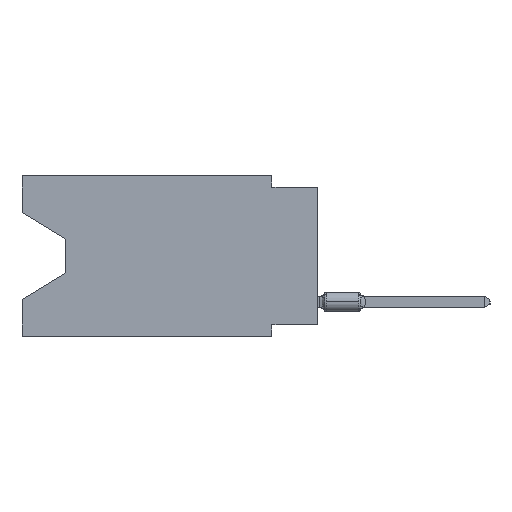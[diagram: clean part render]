
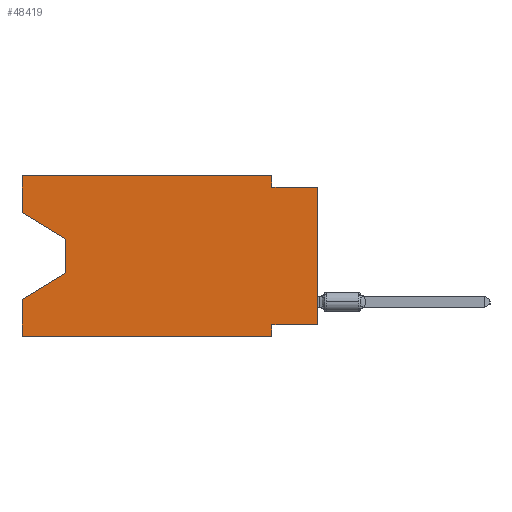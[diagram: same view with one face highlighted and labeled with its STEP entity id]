
A CAD part, left-side view. The second image highlights one B-rep face of the part: STEP entity #48419.
In plain terms, the highlighted planar face has unit normal (-1, 0, 0).
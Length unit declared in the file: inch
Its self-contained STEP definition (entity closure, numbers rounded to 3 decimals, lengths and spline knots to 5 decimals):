
#994 = DIRECTION ( 'NONE',  ( 0., 0., -1. ) ) ;
#1266 = CARTESIAN_POINT ( 'NONE',  ( 0., 0.1, -0.025 ) ) ;
#2979 = LINE ( 'NONE', #18033, #30879 ) ;
#3317 = DIRECTION ( 'NONE',  ( 0., 0.855, -0.519 ) ) ;
#3470 = EDGE_LOOP ( 'NONE', ( #16978, #16556, #7756, #38270, #12181, #52569, #8025, #8264, #33294, #37493, #19391, #17353 ) ) ;
#3641 = EDGE_CURVE ( 'NONE', #18475, #53505, #64559, .T. ) ;
#3717 = CARTESIAN_POINT ( 'NONE',  ( 0., 0.1, 0. ) ) ;
#4876 = CARTESIAN_POINT ( 'NONE',  ( 0., 0.55, -0.138 ) ) ;
#5006 = VECTOR ( 'NONE', #8415, 39.37008 ) ;
#5639 = CARTESIAN_POINT ( 'NONE',  ( 0., 0.645, 0. ) ) ;
#6050 = CARTESIAN_POINT ( 'NONE',  ( 0., 0.645, -0.26975 ) ) ;
#6542 = CARTESIAN_POINT ( 'NONE',  ( 0., 0.645, 0. ) ) ;
#7553 = EDGE_CURVE ( 'NONE', #18475, #38738, #58674, .T. ) ;
#7756 = ORIENTED_EDGE ( 'NONE', *, *, #38244, .T. ) ;
#7978 = EDGE_CURVE ( 'NONE', #9616, #35338, #43878, .T. ) ;
#8025 = ORIENTED_EDGE ( 'NONE', *, *, #7553, .F. ) ;
#8161 = CARTESIAN_POINT ( 'NONE',  ( 0., 0.1, -0.35 ) ) ;
#8264 = ORIENTED_EDGE ( 'NONE', *, *, #3641, .T. ) ;
#8415 = DIRECTION ( 'NONE',  ( 0., 0., 1. ) ) ;
#9101 = VECTOR ( 'NONE', #49989, 39.37008 ) ;
#9375 = DIRECTION ( 'NONE',  ( 0., -0.855, -0.519 ) ) ;
#9616 = VERTEX_POINT ( 'NONE', #64032 ) ;
#10545 = LINE ( 'NONE', #40929, #9101 ) ;
#11681 = LINE ( 'NONE', #22354, #58112 ) ;
#12181 = ORIENTED_EDGE ( 'NONE', *, *, #23631, .T. ) ;
#12814 = VECTOR ( 'NONE', #65021, 39.37008 ) ;
#13101 = AXIS2_PLACEMENT_3D ( 'NONE', #51095, #56427, #35386 ) ;
#14188 = LINE ( 'NONE', #54946, #55352 ) ;
#14520 = DIRECTION ( 'NONE',  ( 0., 0., -1. ) ) ;
#15026 = PLANE ( 'NONE',  #13101 ) ;
#15531 = VERTEX_POINT ( 'NONE', #1266 ) ;
#16556 = ORIENTED_EDGE ( 'NONE', *, *, #31318, .T. ) ;
#16978 = ORIENTED_EDGE ( 'NONE', *, *, #18721, .T. ) ;
#17353 = ORIENTED_EDGE ( 'NONE', *, *, #7978, .F. ) ;
#17809 = VERTEX_POINT ( 'NONE', #3717 ) ;
#18033 = CARTESIAN_POINT ( 'NONE',  ( 0., 0.55, -0.212 ) ) ;
#18475 = VERTEX_POINT ( 'NONE', #20156 ) ;
#18721 = EDGE_CURVE ( 'NONE', #9616, #64779, #44784, .T. ) ;
#19391 = ORIENTED_EDGE ( 'NONE', *, *, #35395, .F. ) ;
#20156 = CARTESIAN_POINT ( 'NONE',  ( 0., 0., -0.325 ) ) ;
#20868 = EDGE_CURVE ( 'NONE', #38738, #26942, #10545, .T. ) ;
#20983 = EDGE_CURVE ( 'NONE', #21154, #50870, #52316, .T. ) ;
#21021 = VECTOR ( 'NONE', #56083, 39.37008 ) ;
#21154 = VERTEX_POINT ( 'NONE', #33531 ) ;
#22354 = CARTESIAN_POINT ( 'NONE',  ( 0., 0.55, -0.138 ) ) ;
#23631 = EDGE_CURVE ( 'NONE', #21154, #26942, #44491, .T. ) ;
#24231 = CARTESIAN_POINT ( 'NONE',  ( 0., 0., -0.325 ) ) ;
#25599 = CARTESIAN_POINT ( 'NONE',  ( 0., 0.1, -0.325 ) ) ;
#26611 = CARTESIAN_POINT ( 'NONE',  ( 0., 0., -0.025 ) ) ;
#26942 = VERTEX_POINT ( 'NONE', #8161 ) ;
#28449 = DIRECTION ( 'NONE',  ( 0., -1., 0. ) ) ;
#30472 = VECTOR ( 'NONE', #32240, 39.37008 ) ;
#30824 = DIRECTION ( 'NONE',  ( 0., 0., 1. ) ) ;
#30879 = VECTOR ( 'NONE', #3317, 39.37008 ) ;
#31318 = EDGE_CURVE ( 'NONE', #64779, #60267, #11681, .T. ) ;
#32240 = DIRECTION ( 'NONE',  ( 0., 0., 1. ) ) ;
#33294 = ORIENTED_EDGE ( 'NONE', *, *, #38813, .F. ) ;
#33531 = CARTESIAN_POINT ( 'NONE',  ( 0., 0.645, -0.35 ) ) ;
#35338 = VERTEX_POINT ( 'NONE', #51091 ) ;
#35386 = DIRECTION ( 'NONE',  ( 0., 0., -1. ) ) ;
#35395 = EDGE_CURVE ( 'NONE', #35338, #17809, #50441, .T. ) ;
#37263 = EDGE_CURVE ( 'NONE', #17809, #15531, #14188, .T. ) ;
#37493 = ORIENTED_EDGE ( 'NONE', *, *, #37263, .F. ) ;
#38244 = EDGE_CURVE ( 'NONE', #60267, #50870, #2979, .T. ) ;
#38270 = ORIENTED_EDGE ( 'NONE', *, *, #20983, .F. ) ;
#38738 = VERTEX_POINT ( 'NONE', #25599 ) ;
#38813 = EDGE_CURVE ( 'NONE', #15531, #53505, #62353, .T. ) ;
#40178 = CARTESIAN_POINT ( 'NONE',  ( 0., 0.645, 0. ) ) ;
#40389 = FACE_OUTER_BOUND ( 'NONE', #3470, .T. ) ;
#40929 = CARTESIAN_POINT ( 'NONE',  ( 0., 0.1, -0.35 ) ) ;
#43453 = CARTESIAN_POINT ( 'NONE',  ( 0., 0.645, -0.08025 ) ) ;
#43740 = VECTOR ( 'NONE', #28449, 39.37008 ) ;
#43878 = LINE ( 'NONE', #40178, #55569 ) ;
#44491 = LINE ( 'NONE', #64907, #44569 ) ;
#44569 = VECTOR ( 'NONE', #49860, 39.37008 ) ;
#44784 = LINE ( 'NONE', #43453, #63489 ) ;
#46625 = CARTESIAN_POINT ( 'NONE',  ( 0., 0., -0.025 ) ) ;
#48419 = ADVANCED_FACE ( 'NONE', ( #40389 ), #15026, .F. ) ;
#49860 = DIRECTION ( 'NONE',  ( 0., -1., 0. ) ) ;
#49989 = DIRECTION ( 'NONE',  ( 0., 0., -1. ) ) ;
#50441 = LINE ( 'NONE', #5639, #21021 ) ;
#50870 = VERTEX_POINT ( 'NONE', #6050 ) ;
#51091 = CARTESIAN_POINT ( 'NONE',  ( 0., 0.645, 0. ) ) ;
#51095 = CARTESIAN_POINT ( 'NONE',  ( 0., 0.645, 0. ) ) ;
#52316 = LINE ( 'NONE', #6542, #30472 ) ;
#52569 = ORIENTED_EDGE ( 'NONE', *, *, #20868, .F. ) ;
#53505 = VERTEX_POINT ( 'NONE', #26611 ) ;
#54946 = CARTESIAN_POINT ( 'NONE',  ( 0., 0.1, 0. ) ) ;
#55352 = VECTOR ( 'NONE', #14520, 39.37008 ) ;
#55569 = VECTOR ( 'NONE', #30824, 39.37008 ) ;
#56083 = DIRECTION ( 'NONE',  ( 0., -1., 0. ) ) ;
#56202 = CARTESIAN_POINT ( 'NONE',  ( 0., 0.55, -0.212 ) ) ;
#56427 = DIRECTION ( 'NONE',  ( 1., 0., 0. ) ) ;
#58112 = VECTOR ( 'NONE', #994, 39.37008 ) ;
#58674 = LINE ( 'NONE', #24231, #12814 ) ;
#60267 = VERTEX_POINT ( 'NONE', #56202 ) ;
#62353 = LINE ( 'NONE', #46625, #43740 ) ;
#63489 = VECTOR ( 'NONE', #9375, 39.37008 ) ;
#64032 = CARTESIAN_POINT ( 'NONE',  ( 0., 0.645, -0.08025 ) ) ;
#64559 = LINE ( 'NONE', #64893, #5006 ) ;
#64779 = VERTEX_POINT ( 'NONE', #4876 ) ;
#64893 = CARTESIAN_POINT ( 'NONE',  ( 0., 0., 0. ) ) ;
#64907 = CARTESIAN_POINT ( 'NONE',  ( 0., 0.645, -0.35 ) ) ;
#65021 = DIRECTION ( 'NONE',  ( 0., 1., 0. ) ) ;
